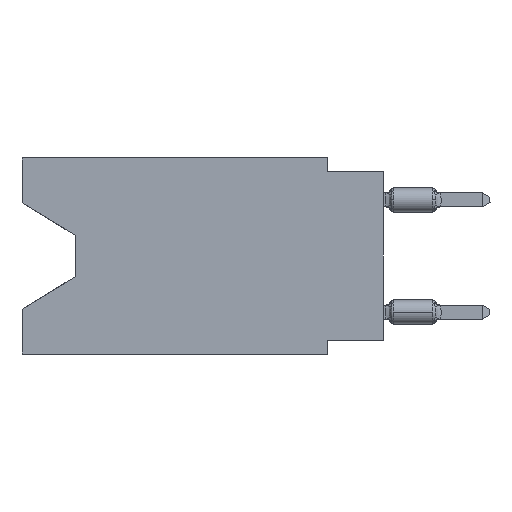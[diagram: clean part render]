
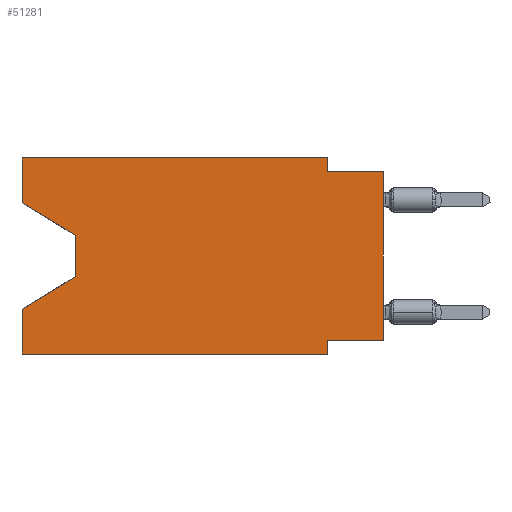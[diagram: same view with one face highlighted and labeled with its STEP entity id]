
A CAD part, left-side view. The second image highlights one B-rep face of the part: STEP entity #51281.
In plain terms, the highlighted planar face has unit normal (-1, 0, 0).
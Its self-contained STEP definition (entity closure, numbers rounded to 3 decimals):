
#413 = ORIENTED_EDGE ( 'NONE', *, *, #3170, .F. ) ;
#1775 = VERTEX_POINT ( 'NONE', #36004 ) ;
#3170 = EDGE_CURVE ( 'NONE', #53736, #42698, #35002, .T. ) ;
#4210 = VECTOR ( 'NONE', #58203, 1000. ) ;
#4224 = EDGE_CURVE ( 'NONE', #34129, #12036, #52666, .T. ) ;
#4310 = DIRECTION ( 'NONE',  ( 0., 1., 0. ) ) ;
#4552 = CARTESIAN_POINT ( 'NONE',  ( 0., 2.54, -0.635 ) ) ;
#4721 = LINE ( 'NONE', #59111, #27167 ) ;
#5559 = EDGE_CURVE ( 'NONE', #44431, #1775, #59350, .T. ) ;
#7734 = CARTESIAN_POINT ( 'NONE',  ( 0., 16.383, -2.038 ) ) ;
#8747 = CARTESIAN_POINT ( 'NONE',  ( 0., 0., -8.255 ) ) ;
#8794 = ORIENTED_EDGE ( 'NONE', *, *, #20900, .F. ) ;
#9124 = LINE ( 'NONE', #15387, #13398 ) ;
#9228 = DIRECTION ( 'NONE',  ( 0., 0., -1. ) ) ;
#9566 = LINE ( 'NONE', #39157, #59606 ) ;
#9648 = DIRECTION ( 'NONE',  ( 0., -1., 0. ) ) ;
#10844 = CARTESIAN_POINT ( 'NONE',  ( 0., 16.383, 0. ) ) ;
#12036 = VERTEX_POINT ( 'NONE', #14162 ) ;
#12104 = CARTESIAN_POINT ( 'NONE',  ( 0., 0., -0.635 ) ) ;
#13291 = ORIENTED_EDGE ( 'NONE', *, *, #36676, .T. ) ;
#13398 = VECTOR ( 'NONE', #13906, 1000. ) ;
#13600 = VERTEX_POINT ( 'NONE', #47948 ) ;
#13731 = CARTESIAN_POINT ( 'NONE',  ( 0., 16.383, 0. ) ) ;
#13906 = DIRECTION ( 'NONE',  ( 0., 0., 1. ) ) ;
#14162 = CARTESIAN_POINT ( 'NONE',  ( 0., 2.54, -8.255 ) ) ;
#14318 = PLANE ( 'NONE',  #53393 ) ;
#14872 = CARTESIAN_POINT ( 'NONE',  ( 0., 2.54, 0. ) ) ;
#15255 = EDGE_LOOP ( 'NONE', ( #25820, #54056, #33365, #17970, #13291, #8794, #20810, #46906, #19352, #28867, #413, #19432 ) ) ;
#15387 = CARTESIAN_POINT ( 'NONE',  ( 0., 0., 0. ) ) ;
#15938 = VERTEX_POINT ( 'NONE', #12104 ) ;
#17970 = ORIENTED_EDGE ( 'NONE', *, *, #26055, .F. ) ;
#18283 = DIRECTION ( 'NONE',  ( 0., 0., -1. ) ) ;
#19352 = ORIENTED_EDGE ( 'NONE', *, *, #31116, .F. ) ;
#19395 = LINE ( 'NONE', #38785, #4210 ) ;
#19432 = ORIENTED_EDGE ( 'NONE', *, *, #52670, .F. ) ;
#20810 = ORIENTED_EDGE ( 'NONE', *, *, #4224, .F. ) ;
#20900 = EDGE_CURVE ( 'NONE', #12036, #45900, #57334, .T. ) ;
#22281 = VECTOR ( 'NONE', #18283, 1000. ) ;
#23869 = VERTEX_POINT ( 'NONE', #4552 ) ;
#25478 = DIRECTION ( 'NONE',  ( 0., -1., 0. ) ) ;
#25820 = ORIENTED_EDGE ( 'NONE', *, *, #5559, .T. ) ;
#26055 = EDGE_CURVE ( 'NONE', #46368, #28476, #4721, .T. ) ;
#26829 = VECTOR ( 'NONE', #9648, 1000. ) ;
#27167 = VECTOR ( 'NONE', #30170, 1000. ) ;
#28476 = VERTEX_POINT ( 'NONE', #45080 ) ;
#28867 = ORIENTED_EDGE ( 'NONE', *, *, #50374, .F. ) ;
#29071 = LINE ( 'NONE', #48453, #26829 ) ;
#30170 = DIRECTION ( 'NONE',  ( 0., 0., 1. ) ) ;
#30740 = VECTOR ( 'NONE', #4310, 1000. ) ;
#31116 = EDGE_CURVE ( 'NONE', #23869, #15938, #19395, .T. ) ;
#31366 = EDGE_CURVE ( 'NONE', #34129, #15938, #9124, .T. ) ;
#31843 = CARTESIAN_POINT ( 'NONE',  ( 0., 13.97, -3.505 ) ) ;
#33231 = LINE ( 'NONE', #61882, #22281 ) ;
#33365 = ORIENTED_EDGE ( 'NONE', *, *, #39219, .T. ) ;
#33467 = CARTESIAN_POINT ( 'NONE',  ( 0., 2.54, -8.89 ) ) ;
#34029 = CARTESIAN_POINT ( 'NONE',  ( 0., 16.383, 0. ) ) ;
#34129 = VERTEX_POINT ( 'NONE', #8747 ) ;
#34650 = FACE_OUTER_BOUND ( 'NONE', #15255, .T. ) ;
#35002 = LINE ( 'NONE', #10844, #38774 ) ;
#35175 = VECTOR ( 'NONE', #60188, 1000. ) ;
#36004 = CARTESIAN_POINT ( 'NONE',  ( 0., 13.97, -3.505 ) ) ;
#36676 = EDGE_CURVE ( 'NONE', #46368, #45900, #29071, .T. ) ;
#38774 = VECTOR ( 'NONE', #25478, 1000. ) ;
#38785 = CARTESIAN_POINT ( 'NONE',  ( 0., 0., -0.635 ) ) ;
#39157 = CARTESIAN_POINT ( 'NONE',  ( 0., 13.97, -5.385 ) ) ;
#39219 = EDGE_CURVE ( 'NONE', #13600, #28476, #9566, .T. ) ;
#40469 = VECTOR ( 'NONE', #45648, 1000. ) ;
#40769 = LINE ( 'NONE', #31843, #35175 ) ;
#41010 = LINE ( 'NONE', #55640, #55745 ) ;
#42698 = VERTEX_POINT ( 'NONE', #14872 ) ;
#44431 = VERTEX_POINT ( 'NONE', #7734 ) ;
#44539 = DIRECTION ( 'NONE',  ( 0., 0.855, -0.519 ) ) ;
#45080 = CARTESIAN_POINT ( 'NONE',  ( 0., 16.383, -6.852 ) ) ;
#45648 = DIRECTION ( 'NONE',  ( 0., -0.855, -0.519 ) ) ;
#45900 = VERTEX_POINT ( 'NONE', #56518 ) ;
#46242 = VECTOR ( 'NONE', #47146, 1000. ) ;
#46368 = VERTEX_POINT ( 'NONE', #62489 ) ;
#46906 = ORIENTED_EDGE ( 'NONE', *, *, #31366, .T. ) ;
#47146 = DIRECTION ( 'NONE',  ( 0., 0., -1. ) ) ;
#47894 = CARTESIAN_POINT ( 'NONE',  ( 0., 0., -8.255 ) ) ;
#47948 = CARTESIAN_POINT ( 'NONE',  ( 0., 13.97, -5.385 ) ) ;
#48453 = CARTESIAN_POINT ( 'NONE',  ( 0., 16.383, -8.89 ) ) ;
#49286 = DIRECTION ( 'NONE',  ( 1., 0., 0. ) ) ;
#50374 = EDGE_CURVE ( 'NONE', #42698, #23869, #33231, .T. ) ;
#51281 = ADVANCED_FACE ( 'NONE', ( #34650 ), #14318, .F. ) ;
#52229 = EDGE_CURVE ( 'NONE', #1775, #13600, #40769, .T. ) ;
#52666 = LINE ( 'NONE', #47894, #30740 ) ;
#52670 = EDGE_CURVE ( 'NONE', #44431, #53736, #41010, .T. ) ;
#53393 = AXIS2_PLACEMENT_3D ( 'NONE', #34029, #49286, #9228 ) ;
#53736 = VERTEX_POINT ( 'NONE', #13731 ) ;
#54056 = ORIENTED_EDGE ( 'NONE', *, *, #52229, .T. ) ;
#54703 = DIRECTION ( 'NONE',  ( 0., 0., 1. ) ) ;
#55640 = CARTESIAN_POINT ( 'NONE',  ( 0., 16.383, 0. ) ) ;
#55745 = VECTOR ( 'NONE', #54703, 1000. ) ;
#55824 = CARTESIAN_POINT ( 'NONE',  ( 0., 16.383, -2.038 ) ) ;
#56518 = CARTESIAN_POINT ( 'NONE',  ( 0., 2.54, -8.89 ) ) ;
#57334 = LINE ( 'NONE', #33467, #46242 ) ;
#58203 = DIRECTION ( 'NONE',  ( 0., -1., 0. ) ) ;
#59111 = CARTESIAN_POINT ( 'NONE',  ( 0., 16.383, 0. ) ) ;
#59350 = LINE ( 'NONE', #55824, #40469 ) ;
#59606 = VECTOR ( 'NONE', #44539, 1000. ) ;
#60188 = DIRECTION ( 'NONE',  ( 0., 0., -1. ) ) ;
#61882 = CARTESIAN_POINT ( 'NONE',  ( 0., 2.54, 0. ) ) ;
#62489 = CARTESIAN_POINT ( 'NONE',  ( 0., 16.383, -8.89 ) ) ;
